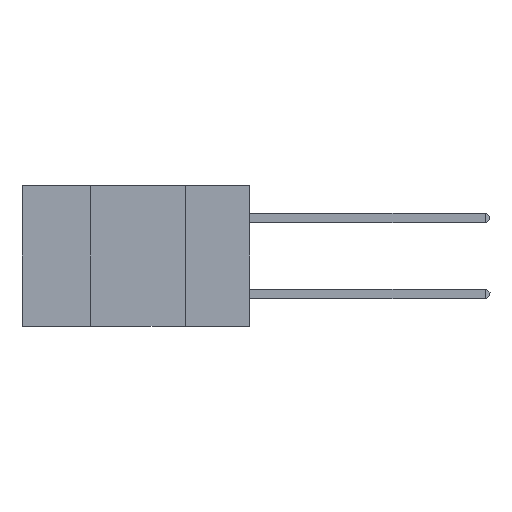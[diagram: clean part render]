
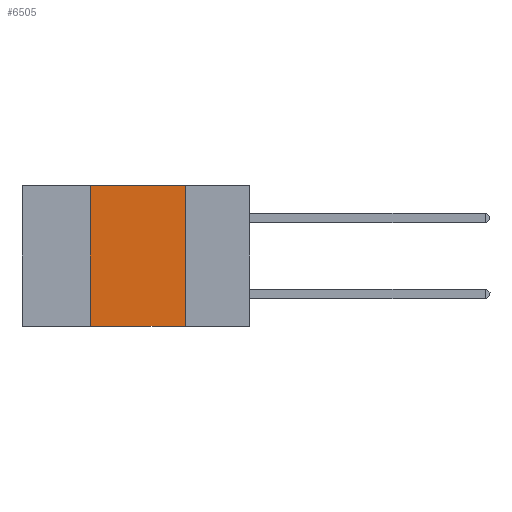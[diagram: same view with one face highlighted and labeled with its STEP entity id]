
A CAD part, left-side view. The second image highlights one B-rep face of the part: STEP entity #6505.
In plain terms, the highlighted planar face has unit normal (-1, 0, 0).
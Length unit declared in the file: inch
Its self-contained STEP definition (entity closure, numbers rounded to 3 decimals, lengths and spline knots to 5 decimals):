
#198 = CARTESIAN_POINT ( 'NONE',  ( 0., 0.17, -0.37 ) ) ;
#844 = VECTOR ( 'NONE', #3696, 39.37008 ) ;
#998 = CARTESIAN_POINT ( 'NONE',  ( 0., 0.6, -0.37 ) ) ;
#1110 = LINE ( 'NONE', #998, #844 ) ;
#1588 = DIRECTION ( 'NONE',  ( 0., 0., -1. ) ) ;
#1827 = ORIENTED_EDGE ( 'NONE', *, *, #2243, .F. ) ;
#2243 = EDGE_CURVE ( 'NONE', #3116, #7910, #10121, .T. ) ;
#2541 = VECTOR ( 'NONE', #3267, 39.37008 ) ;
#2713 = VECTOR ( 'NONE', #1588, 39.37008 ) ;
#3108 = EDGE_CURVE ( 'NONE', #7910, #9198, #5079, .T. ) ;
#3116 = VERTEX_POINT ( 'NONE', #6793 ) ;
#3195 = CARTESIAN_POINT ( 'NONE',  ( 0., 0.42, 0. ) ) ;
#3267 = DIRECTION ( 'NONE',  ( 0., 0., 1. ) ) ;
#3696 = DIRECTION ( 'NONE',  ( 0., -1., 0. ) ) ;
#5050 = DIRECTION ( 'NONE',  ( 1., 0., 0. ) ) ;
#5079 = LINE ( 'NONE', #7687, #2713 ) ;
#5196 = CARTESIAN_POINT ( 'NONE',  ( 0., 0.42, -0.37 ) ) ;
#5241 = VERTEX_POINT ( 'NONE', #5196 ) ;
#6077 = VECTOR ( 'NONE', #11431, 39.37008 ) ;
#6505 = ADVANCED_FACE ( 'NONE', ( #9899 ), #10369, .F. ) ;
#6778 = ORIENTED_EDGE ( 'NONE', *, *, #9833, .T. ) ;
#6793 = CARTESIAN_POINT ( 'NONE',  ( 0., 0.42, 0. ) ) ;
#7090 = ORIENTED_EDGE ( 'NONE', *, *, #3108, .F. ) ;
#7610 = EDGE_LOOP ( 'NONE', ( #7090, #1827, #9645, #6778 ) ) ;
#7687 = CARTESIAN_POINT ( 'NONE',  ( 0., 0.17, 0. ) ) ;
#7837 = CARTESIAN_POINT ( 'NONE',  ( 0., 0.6, 0. ) ) ;
#7910 = VERTEX_POINT ( 'NONE', #10220 ) ;
#8677 = EDGE_CURVE ( 'NONE', #5241, #3116, #8795, .T. ) ;
#8795 = LINE ( 'NONE', #3195, #2541 ) ;
#9198 = VERTEX_POINT ( 'NONE', #198 ) ;
#9645 = ORIENTED_EDGE ( 'NONE', *, *, #8677, .F. ) ;
#9833 = EDGE_CURVE ( 'NONE', #5241, #9198, #1110, .T. ) ;
#9899 = FACE_OUTER_BOUND ( 'NONE', #7610, .T. ) ;
#10121 = LINE ( 'NONE', #7837, #6077 ) ;
#10220 = CARTESIAN_POINT ( 'NONE',  ( 0., 0.17, 0. ) ) ;
#10369 = PLANE ( 'NONE',  #10631 ) ;
#10631 = AXIS2_PLACEMENT_3D ( 'NONE', #11153, #5050, #11259 ) ;
#11153 = CARTESIAN_POINT ( 'NONE',  ( 0., 0.6, 0. ) ) ;
#11259 = DIRECTION ( 'NONE',  ( 0., 0., -1. ) ) ;
#11431 = DIRECTION ( 'NONE',  ( 0., -1., 0. ) ) ;
